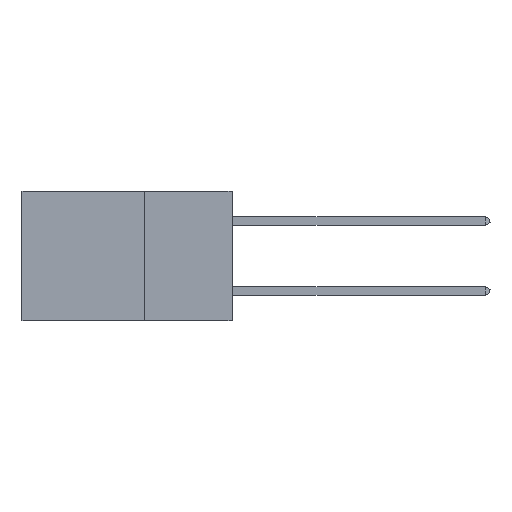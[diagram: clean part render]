
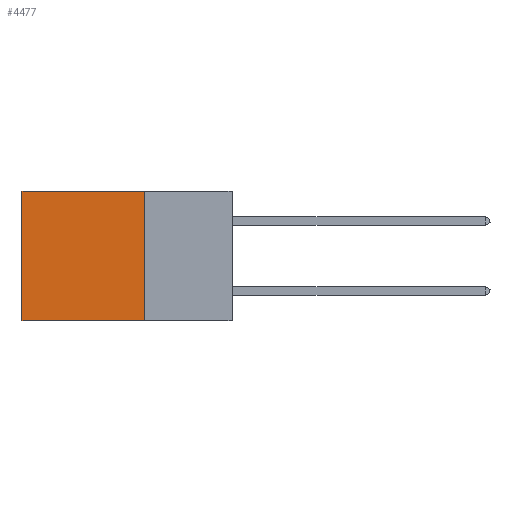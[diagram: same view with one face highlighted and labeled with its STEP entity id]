
A CAD part, left-side view. The second image highlights one B-rep face of the part: STEP entity #4477.
In plain terms, the highlighted planar face has unit normal (-1, 0, 0).
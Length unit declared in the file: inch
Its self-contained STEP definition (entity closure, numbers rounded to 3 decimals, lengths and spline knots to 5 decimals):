
#1461 = DIRECTION ( 'NONE',  ( 0., 1., 0. ) ) ;
#2648 = VERTEX_POINT ( 'NONE', #17369 ) ;
#2773 = ORIENTED_EDGE ( 'NONE', *, *, #16423, .F. ) ;
#3479 = EDGE_LOOP ( 'NONE', ( #18748, #5959, #2773, #4256 ) ) ;
#4193 = DIRECTION ( 'NONE',  ( 0., 0., -1. ) ) ;
#4256 = ORIENTED_EDGE ( 'NONE', *, *, #12284, .T. ) ;
#4273 = DIRECTION ( 'NONE',  ( 1., 0., 0. ) ) ;
#4349 = VERTEX_POINT ( 'NONE', #8608 ) ;
#4415 = PLANE ( 'NONE',  #17850 ) ;
#4477 = ADVANCED_FACE ( 'NONE', ( #18155 ), #4415, .F. ) ;
#4604 = CARTESIAN_POINT ( 'NONE',  ( 0.2875, 0.25, 0. ) ) ;
#5534 = DIRECTION ( 'NONE',  ( 0., 0., -1. ) ) ;
#5959 = ORIENTED_EDGE ( 'NONE', *, *, #11001, .F. ) ;
#7595 = VECTOR ( 'NONE', #1461, 39.37008 ) ;
#8386 = VECTOR ( 'NONE', #18776, 39.37008 ) ;
#8608 = CARTESIAN_POINT ( 'NONE',  ( 0.2875, 0.25, -0.37 ) ) ;
#8926 = VERTEX_POINT ( 'NONE', #10832 ) ;
#9040 = CARTESIAN_POINT ( 'NONE',  ( 0.2875, 0.6, 0. ) ) ;
#9658 = CARTESIAN_POINT ( 'NONE',  ( 0.2875, 0.25, 0. ) ) ;
#9826 = CARTESIAN_POINT ( 'NONE',  ( 0.2875, 0.25, -0.37 ) ) ;
#10832 = CARTESIAN_POINT ( 'NONE',  ( 0.2875, 0.6, 0. ) ) ;
#11001 = EDGE_CURVE ( 'NONE', #4349, #11243, #15253, .T. ) ;
#11243 = VERTEX_POINT ( 'NONE', #16824 ) ;
#11262 = VECTOR ( 'NONE', #5534, 39.37008 ) ;
#12284 = EDGE_CURVE ( 'NONE', #2648, #8926, #16702, .T. ) ;
#12779 = LINE ( 'NONE', #9040, #8386 ) ;
#13754 = CARTESIAN_POINT ( 'NONE',  ( 0.2875, 0.25, 0. ) ) ;
#14590 = DIRECTION ( 'NONE',  ( 0., 1., 0. ) ) ;
#15253 = LINE ( 'NONE', #9826, #7595 ) ;
#16423 = EDGE_CURVE ( 'NONE', #2648, #4349, #19844, .T. ) ;
#16477 = VECTOR ( 'NONE', #14590, 39.37008 ) ;
#16702 = LINE ( 'NONE', #9658, #16477 ) ;
#16824 = CARTESIAN_POINT ( 'NONE',  ( 0.2875, 0.6, -0.37 ) ) ;
#17228 = EDGE_CURVE ( 'NONE', #8926, #11243, #12779, .T. ) ;
#17369 = CARTESIAN_POINT ( 'NONE',  ( 0.2875, 0.25, 0. ) ) ;
#17850 = AXIS2_PLACEMENT_3D ( 'NONE', #4604, #4273, #4193 ) ;
#18155 = FACE_OUTER_BOUND ( 'NONE', #3479, .T. ) ;
#18748 = ORIENTED_EDGE ( 'NONE', *, *, #17228, .T. ) ;
#18776 = DIRECTION ( 'NONE',  ( 0., 0., -1. ) ) ;
#19844 = LINE ( 'NONE', #13754, #11262 ) ;
